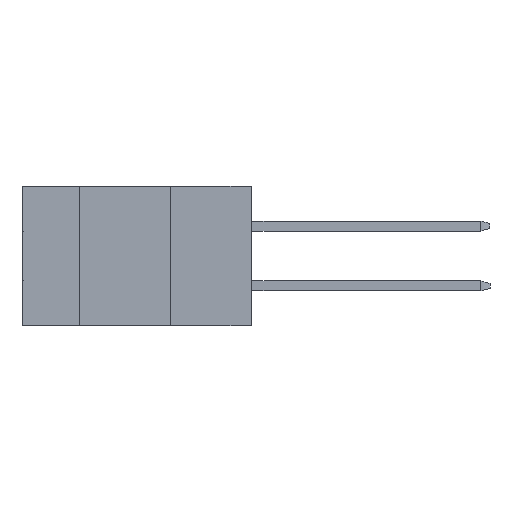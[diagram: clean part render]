
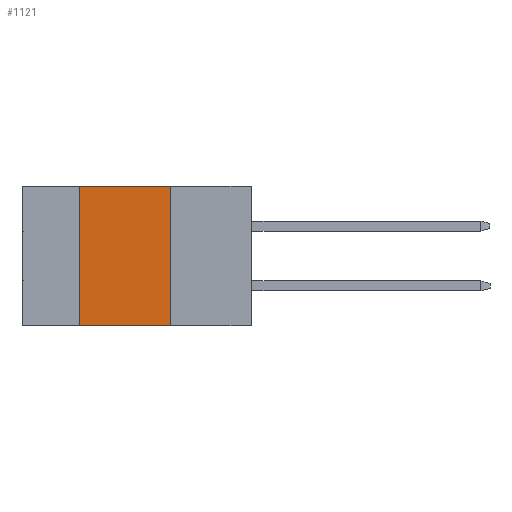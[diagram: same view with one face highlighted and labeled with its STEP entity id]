
A CAD part, left-side view. The second image highlights one B-rep face of the part: STEP entity #1121.
In plain terms, the highlighted planar face has unit normal (-1, 0, 0).
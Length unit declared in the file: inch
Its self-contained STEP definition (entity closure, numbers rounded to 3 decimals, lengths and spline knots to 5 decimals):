
#491 = DIRECTION ( 'NONE',  ( 0., 0., -1. ) ) ;
#593 = CARTESIAN_POINT ( 'NONE',  ( 0., 0.72, 0. ) ) ;
#638 = EDGE_CURVE ( 'NONE', #22295, #18816, #19633, .T. ) ;
#906 = LINE ( 'NONE', #2523, #8593 ) ;
#1121 = ADVANCED_FACE ( 'NONE', ( #21440 ), #9215, .F. ) ;
#1655 = VERTEX_POINT ( 'NONE', #5696 ) ;
#1682 = EDGE_CURVE ( 'NONE', #18816, #1655, #11219, .T. ) ;
#2523 = CARTESIAN_POINT ( 'NONE',  ( 0., 0.54, -0.437 ) ) ;
#5696 = CARTESIAN_POINT ( 'NONE',  ( 0., 0.254, -0.437 ) ) ;
#5814 = DIRECTION ( 'NONE',  ( 0., 0., -1. ) ) ;
#7551 = CARTESIAN_POINT ( 'NONE',  ( 0., 0.254, -0.437 ) ) ;
#8593 = VECTOR ( 'NONE', #16565, 39.37008 ) ;
#9030 = VECTOR ( 'NONE', #16063, 39.37008 ) ;
#9215 = PLANE ( 'NONE',  #18527 ) ;
#9679 = ORIENTED_EDGE ( 'NONE', *, *, #12313, .T. ) ;
#10007 = ORIENTED_EDGE ( 'NONE', *, *, #21366, .F. ) ;
#11219 = LINE ( 'NONE', #7551, #13843 ) ;
#12313 = EDGE_CURVE ( 'NONE', #17363, #1655, #17803, .T. ) ;
#12896 = DIRECTION ( 'NONE',  ( 1., 0., 0. ) ) ;
#13292 = ORIENTED_EDGE ( 'NONE', *, *, #638, .F. ) ;
#13843 = VECTOR ( 'NONE', #5814, 39.37008 ) ;
#14441 = CARTESIAN_POINT ( 'NONE',  ( 0., 0.72, 0. ) ) ;
#15348 = CARTESIAN_POINT ( 'NONE',  ( 0., 0.54, 0. ) ) ;
#16063 = DIRECTION ( 'NONE',  ( 0., -1., 0. ) ) ;
#16123 = EDGE_LOOP ( 'NONE', ( #20453, #13292, #10007, #9679 ) ) ;
#16565 = DIRECTION ( 'NONE',  ( 0., 0., 1. ) ) ;
#17363 = VERTEX_POINT ( 'NONE', #21671 ) ;
#17694 = DIRECTION ( 'NONE',  ( 0., -1., 0. ) ) ;
#17803 = LINE ( 'NONE', #21381, #21686 ) ;
#18527 = AXIS2_PLACEMENT_3D ( 'NONE', #593, #12896, #491 ) ;
#18816 = VERTEX_POINT ( 'NONE', #20177 ) ;
#19633 = LINE ( 'NONE', #14441, #9030 ) ;
#20177 = CARTESIAN_POINT ( 'NONE',  ( 0., 0.254, 0. ) ) ;
#20453 = ORIENTED_EDGE ( 'NONE', *, *, #1682, .F. ) ;
#21366 = EDGE_CURVE ( 'NONE', #17363, #22295, #906, .T. ) ;
#21381 = CARTESIAN_POINT ( 'NONE',  ( 0., 0.72, -0.437 ) ) ;
#21440 = FACE_OUTER_BOUND ( 'NONE', #16123, .T. ) ;
#21671 = CARTESIAN_POINT ( 'NONE',  ( 0., 0.54, -0.437 ) ) ;
#21686 = VECTOR ( 'NONE', #17694, 39.37008 ) ;
#22295 = VERTEX_POINT ( 'NONE', #15348 ) ;
